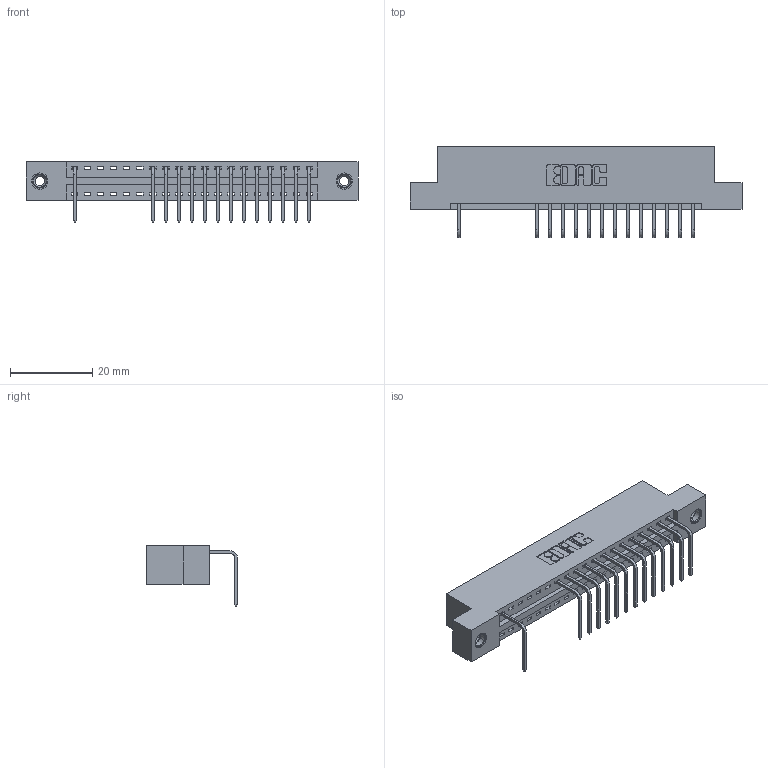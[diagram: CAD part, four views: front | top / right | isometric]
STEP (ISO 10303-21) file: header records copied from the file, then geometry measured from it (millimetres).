
FILE_DESCRIPTION (( 'STEP AP203' ), '1' );
FILE_NAME ('346-019-558-108.STEP', '2018-08-20T10:25:09', ( '' ), ( '' ), 'SwSTEP 2.0', 'SolidWorks 2016', '' );
FILE_SCHEMA (( 'CONFIG_CONTROL_DESIGN' ));
Length unit declared in the file: inch
Products named in the file (4): 346 Part_Flush Mounting Lugs - 0.156 Dia-TI; 345-292-001_558 Tail - 2; 345-250-001_345-250-003-102; 346-019-558-108
Assembly tree (17 placements, depth 2):
  346-019-558-108
    346 Part_Flush Mounting Lugs - 0.156 Dia-TI
    345-292-001_558 Tail - 2  x14
    345-250-001_345-250-003-102  x2
Bounding box: 80.9 x 22.16 x 14.73 mm (x, y, z)
Volume: 7568.3 mm3; surface area: 9203.6 mm2
Topology: 17 solids, 17 shells, 1082 faces, 3223 edges, 2122 vertices
Faces by surface type: plane 746, cylinder 320, cone 12, torus 4
Entity records: 15998 total; most frequent: CARTESIAN_POINT 2755, ORIENTED_EDGE 2706, DIRECTION 2479, EDGE_CURVE 1353, VECTOR 1125, LINE 1125, VERTEX_POINT 896, AXIS2_PLACEMENT_3D 677
